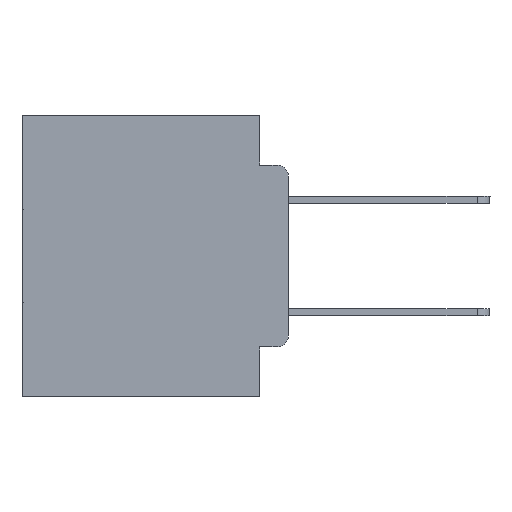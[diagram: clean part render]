
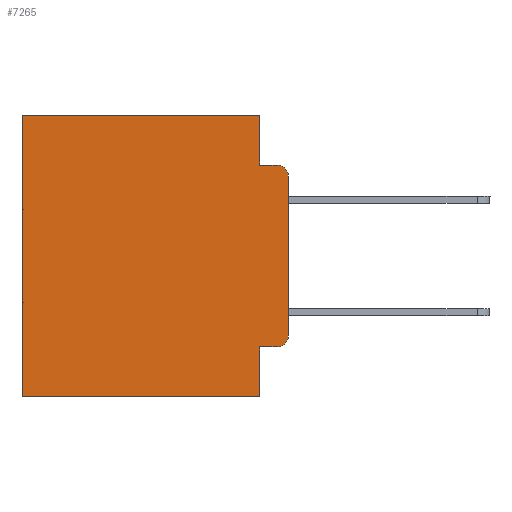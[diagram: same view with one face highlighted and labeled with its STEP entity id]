
A CAD part, left-side view. The second image highlights one B-rep face of the part: STEP entity #7265.
In plain terms, the highlighted planar face has unit normal (-1, 0, 0).
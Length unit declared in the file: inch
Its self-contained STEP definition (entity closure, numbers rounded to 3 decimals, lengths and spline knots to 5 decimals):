
#707 = EDGE_CURVE ( 'NONE', #11502, #13832, #28607, .T. ) ;
#779 = ORIENTED_EDGE ( 'NONE', *, *, #707, .T. ) ;
#1141 = VERTEX_POINT ( 'NONE', #30455 ) ;
#1278 = CARTESIAN_POINT ( 'NONE',  ( 0.298, 0., -0.1085 ) ) ;
#1350 = CARTESIAN_POINT ( 'NONE',  ( 0.298, 0.051, -0.0885 ) ) ;
#2040 = DIRECTION ( 'NONE',  ( 0., 0., -1. ) ) ;
#2182 = DIRECTION ( 'NONE',  ( 0., 0., -1. ) ) ;
#2327 = EDGE_CURVE ( 'NONE', #28520, #1141, #9095, .T. ) ;
#2995 = CARTESIAN_POINT ( 'NONE',  ( 0.298, 0.051, 0. ) ) ;
#3101 = CARTESIAN_POINT ( 'NONE',  ( 0.298, 0.02, -0.0885 ) ) ;
#3264 = ORIENTED_EDGE ( 'NONE', *, *, #7757, .F. ) ;
#3889 = CARTESIAN_POINT ( 'NONE',  ( 0.298, 0.051, -0.0885 ) ) ;
#3912 = EDGE_CURVE ( 'NONE', #28520, #28007, #16816, .T. ) ;
#4509 = DIRECTION ( 'NONE',  ( 0., -1., 0. ) ) ;
#4534 = CARTESIAN_POINT ( 'NONE',  ( 0.298, 0.051, -0.4115 ) ) ;
#4537 = VERTEX_POINT ( 'NONE', #21331 ) ;
#4847 = DIRECTION ( 'NONE',  ( -1., 0., 0. ) ) ;
#5405 = DIRECTION ( 'NONE',  ( 0., 0., -1. ) ) ;
#5447 = VECTOR ( 'NONE', #22031, 39.37008 ) ;
#5956 = DIRECTION ( 'NONE',  ( 1., 0., 0. ) ) ;
#6940 = LINE ( 'NONE', #16343, #24997 ) ;
#7012 = PLANE ( 'NONE',  #23156 ) ;
#7258 = ORIENTED_EDGE ( 'NONE', *, *, #10310, .T. ) ;
#7265 = ADVANCED_FACE ( 'NONE', ( #7745 ), #7012, .F. ) ;
#7745 = FACE_OUTER_BOUND ( 'NONE', #17031, .T. ) ;
#7757 = EDGE_CURVE ( 'NONE', #19569, #24444, #30357, .T. ) ;
#8360 = VECTOR ( 'NONE', #16665, 39.37008 ) ;
#8726 = CARTESIAN_POINT ( 'NONE',  ( 0.298, 0.02, -0.4115 ) ) ;
#9095 = LINE ( 'NONE', #14682, #8360 ) ;
#9828 = LINE ( 'NONE', #3889, #22397 ) ;
#10121 = ORIENTED_EDGE ( 'NONE', *, *, #17311, .T. ) ;
#10310 = EDGE_CURVE ( 'NONE', #28007, #24444, #10788, .T. ) ;
#10587 = CIRCLE ( 'NONE', #18249, 0.02 ) ;
#10788 = CIRCLE ( 'NONE', #13953, 0.02 ) ;
#10836 = EDGE_CURVE ( 'NONE', #4537, #11502, #27995, .T. ) ;
#10893 = CARTESIAN_POINT ( 'NONE',  ( 0.298, 0.473, -0.5 ) ) ;
#11134 = VERTEX_POINT ( 'NONE', #1350 ) ;
#11502 = VERTEX_POINT ( 'NONE', #23930 ) ;
#12109 = ORIENTED_EDGE ( 'NONE', *, *, #13982, .F. ) ;
#12295 = ORIENTED_EDGE ( 'NONE', *, *, #3912, .T. ) ;
#12954 = CARTESIAN_POINT ( 'NONE',  ( 0.298, 0.051, -0.4115 ) ) ;
#13387 = DIRECTION ( 'NONE',  ( 0., -1., 0. ) ) ;
#13832 = VERTEX_POINT ( 'NONE', #10893 ) ;
#13953 = AXIS2_PLACEMENT_3D ( 'NONE', #19094, #4847, #21456 ) ;
#13982 = EDGE_CURVE ( 'NONE', #1141, #13832, #6940, .T. ) ;
#14017 = DIRECTION ( 'NONE',  ( 0., 1., 0. ) ) ;
#14682 = CARTESIAN_POINT ( 'NONE',  ( 0.298, 0.051, 0. ) ) ;
#15675 = VECTOR ( 'NONE', #5405, 39.37008 ) ;
#15763 = ORIENTED_EDGE ( 'NONE', *, *, #23564, .F. ) ;
#16340 = DIRECTION ( 'NONE',  ( -1., 0., 0. ) ) ;
#16343 = CARTESIAN_POINT ( 'NONE',  ( 0.298, 0., -0.5 ) ) ;
#16392 = VECTOR ( 'NONE', #14017, 39.37008 ) ;
#16510 = CARTESIAN_POINT ( 'NONE',  ( 0.298, 0.473, 0. ) ) ;
#16665 = DIRECTION ( 'NONE',  ( 0., 0., -1. ) ) ;
#16816 = LINE ( 'NONE', #4534, #17555 ) ;
#17031 = EDGE_LOOP ( 'NONE', ( #3264, #10121, #15763, #19411, #20426, #779, #12109, #18998, #12295, #7258 ) ) ;
#17311 = EDGE_CURVE ( 'NONE', #19569, #26010, #10587, .T. ) ;
#17555 = VECTOR ( 'NONE', #4509, 39.37008 ) ;
#18249 = AXIS2_PLACEMENT_3D ( 'NONE', #30180, #16340, #2040 ) ;
#18998 = ORIENTED_EDGE ( 'NONE', *, *, #2327, .F. ) ;
#19094 = CARTESIAN_POINT ( 'NONE',  ( 0.298, 0.02, -0.3915 ) ) ;
#19411 = ORIENTED_EDGE ( 'NONE', *, *, #25108, .F. ) ;
#19546 = DIRECTION ( 'NONE',  ( 0., 0., -1. ) ) ;
#19569 = VERTEX_POINT ( 'NONE', #1278 ) ;
#19780 = CARTESIAN_POINT ( 'NONE',  ( 0.298, 0., 0. ) ) ;
#20426 = ORIENTED_EDGE ( 'NONE', *, *, #10836, .T. ) ;
#21331 = CARTESIAN_POINT ( 'NONE',  ( 0.298, 0.051, 0. ) ) ;
#21456 = DIRECTION ( 'NONE',  ( 0., 0., -1. ) ) ;
#22031 = DIRECTION ( 'NONE',  ( 0., 0., -1. ) ) ;
#22397 = VECTOR ( 'NONE', #13387, 39.37008 ) ;
#23156 = AXIS2_PLACEMENT_3D ( 'NONE', #24019, #5956, #2182 ) ;
#23564 = EDGE_CURVE ( 'NONE', #11134, #26010, #9828, .T. ) ;
#23930 = CARTESIAN_POINT ( 'NONE',  ( 0.298, 0.473, 0. ) ) ;
#24019 = CARTESIAN_POINT ( 'NONE',  ( 0.298, 0., 0. ) ) ;
#24444 = VERTEX_POINT ( 'NONE', #28343 ) ;
#24997 = VECTOR ( 'NONE', #30184, 39.37008 ) ;
#25108 = EDGE_CURVE ( 'NONE', #4537, #11134, #28033, .T. ) ;
#26010 = VERTEX_POINT ( 'NONE', #3101 ) ;
#27959 = CARTESIAN_POINT ( 'NONE',  ( 0.298, 0., 0. ) ) ;
#27995 = LINE ( 'NONE', #27959, #16392 ) ;
#28007 = VERTEX_POINT ( 'NONE', #8726 ) ;
#28033 = LINE ( 'NONE', #2995, #15675 ) ;
#28343 = CARTESIAN_POINT ( 'NONE',  ( 0.298, 0., -0.3915 ) ) ;
#28520 = VERTEX_POINT ( 'NONE', #12954 ) ;
#28607 = LINE ( 'NONE', #16510, #29322 ) ;
#29322 = VECTOR ( 'NONE', #19546, 39.37008 ) ;
#30180 = CARTESIAN_POINT ( 'NONE',  ( 0.298, 0.02, -0.1085 ) ) ;
#30184 = DIRECTION ( 'NONE',  ( 0., 1., 0. ) ) ;
#30357 = LINE ( 'NONE', #19780, #5447 ) ;
#30455 = CARTESIAN_POINT ( 'NONE',  ( 0.298, 0.051, -0.5 ) ) ;
